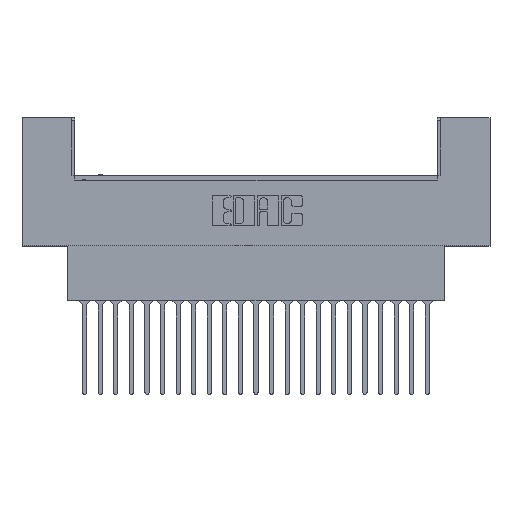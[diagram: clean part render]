
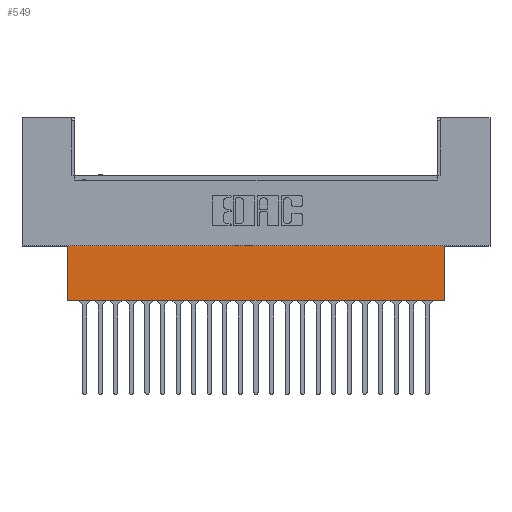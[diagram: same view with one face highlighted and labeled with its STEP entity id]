
A CAD part, top view. The second image highlights one B-rep face of the part: STEP entity #549.
In plain terms, the highlighted planar face has unit normal (0, 0, 1).
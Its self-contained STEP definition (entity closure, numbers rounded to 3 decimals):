
#549 = ADVANCED_FACE ( 'NONE', ( #19171 ), #1168, .F. ) ;
#1168 = PLANE ( 'NONE',  #15601 ) ;
#3177 = DIRECTION ( 'NONE',  ( 0., 1., 0. ) ) ;
#3555 = CARTESIAN_POINT ( 'NONE',  ( 68.885, -8.814, -3.962 ) ) ;
#3563 = VECTOR ( 'NONE', #10244, 1000. ) ;
#4380 = CARTESIAN_POINT ( 'NONE',  ( 68.885, 0., -3.962 ) ) ;
#5491 = EDGE_CURVE ( 'NONE', #9676, #18083, #23078, .T. ) ;
#6449 = DIRECTION ( 'NONE',  ( -1., 0., 0. ) ) ;
#7884 = LINE ( 'NONE', #21370, #3563 ) ;
#8731 = CARTESIAN_POINT ( 'NONE',  ( 76.352, -8.814, -3.962 ) ) ;
#9676 = VERTEX_POINT ( 'NONE', #4380 ) ;
#9758 = CARTESIAN_POINT ( 'NONE',  ( 7.468, 0., -3.962 ) ) ;
#10118 = CARTESIAN_POINT ( 'NONE',  ( 76.352, 0., -3.962 ) ) ;
#10244 = DIRECTION ( 'NONE',  ( 0., 1., 0. ) ) ;
#10296 = LINE ( 'NONE', #27772, #23974 ) ;
#10700 = DIRECTION ( 'NONE',  ( -1., 0., 0. ) ) ;
#13554 = ORIENTED_EDGE ( 'NONE', *, *, #5491, .T. ) ;
#14473 = EDGE_LOOP ( 'NONE', ( #25713, #18498, #13554, #22676 ) ) ;
#14783 = LINE ( 'NONE', #8731, #28116 ) ;
#15601 = AXIS2_PLACEMENT_3D ( 'NONE', #10118, #17229, #3177 ) ;
#17229 = DIRECTION ( 'NONE',  ( 0., 0., -1. ) ) ;
#17512 = CARTESIAN_POINT ( 'NONE',  ( 76.352, 0., -3.962 ) ) ;
#18083 = VERTEX_POINT ( 'NONE', #9758 ) ;
#18404 = EDGE_CURVE ( 'NONE', #24421, #23653, #14783, .T. ) ;
#18498 = ORIENTED_EDGE ( 'NONE', *, *, #24826, .F. ) ;
#19171 = FACE_OUTER_BOUND ( 'NONE', #14473, .T. ) ;
#19830 = EDGE_CURVE ( 'NONE', #23653, #18083, #7884, .T. ) ;
#20767 = DIRECTION ( 'NONE',  ( 0., -1., 0. ) ) ;
#21370 = CARTESIAN_POINT ( 'NONE',  ( 7.468, -8.814, -3.962 ) ) ;
#22676 = ORIENTED_EDGE ( 'NONE', *, *, #19830, .F. ) ;
#23078 = LINE ( 'NONE', #17512, #26720 ) ;
#23653 = VERTEX_POINT ( 'NONE', #25833 ) ;
#23974 = VECTOR ( 'NONE', #20767, 1000. ) ;
#24421 = VERTEX_POINT ( 'NONE', #3555 ) ;
#24826 = EDGE_CURVE ( 'NONE', #9676, #24421, #10296, .T. ) ;
#25713 = ORIENTED_EDGE ( 'NONE', *, *, #18404, .F. ) ;
#25833 = CARTESIAN_POINT ( 'NONE',  ( 7.468, -8.814, -3.962 ) ) ;
#26720 = VECTOR ( 'NONE', #10700, 1000. ) ;
#27772 = CARTESIAN_POINT ( 'NONE',  ( 68.885, -8.814, -3.962 ) ) ;
#28116 = VECTOR ( 'NONE', #6449, 1000. ) ;
